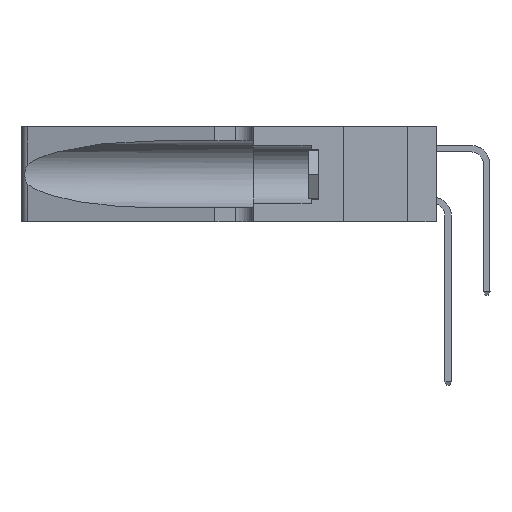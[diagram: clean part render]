
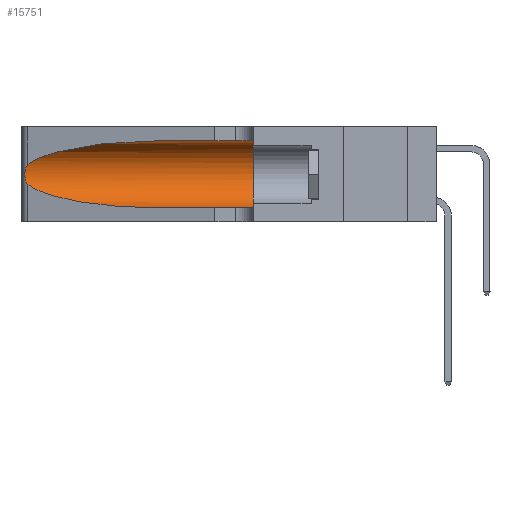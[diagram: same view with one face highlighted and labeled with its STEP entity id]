
A CAD part, left-side view. The second image highlights one B-rep face of the part: STEP entity #15751.
In plain terms, the highlighted cylindrical face has radius 3.308 mm (diameter 6.617 mm), a partial arc.
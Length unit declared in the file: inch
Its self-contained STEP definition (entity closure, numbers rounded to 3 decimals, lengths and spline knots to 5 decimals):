
#18 = DIRECTION ( 'NONE',  ( 0., -1., 0. ) ) ;
#241 = CARTESIAN_POINT ( 'NONE',  ( 0.1305, 0.35, 0.31525 ) ) ;
#1112 = ORIENTED_EDGE ( 'NONE', *, *, #20133, .T. ) ;
#1433 = VERTEX_POINT ( 'NONE', #8854 ) ;
#1655 = CARTESIAN_POINT ( 'NONE',  ( 0.25639, 1.23184, 0.21858 ) ) ;
#2651 = CARTESIAN_POINT ( 'NONE',  ( 0.1305, 0.35, 0.05475 ) ) ;
#3214 =( BOUNDED_CURVE ( )  B_SPLINE_CURVE ( 3, ( #38986, #42524, #31721, #24974 ),
 .UNSPECIFIED., .F., .F. ) 
 B_SPLINE_CURVE_WITH_KNOTS ( ( 4, 4 ),
 ( 1.5708, 2.84003 ),
 .UNSPECIFIED. ) 
 CURVE ( )  GEOMETRIC_REPRESENTATION_ITEM ( )  RATIONAL_B_SPLINE_CURVE ( ( 1., 0.87, 0.87, 1. ) ) 
 REPRESENTATION_ITEM ( '' )  );
#3647 = CARTESIAN_POINT ( 'NONE',  ( 0.1305, 1.61858, 0.185 ) ) ;
#5121 = VERTEX_POINT ( 'NONE', #241 ) ;
#5145 = EDGE_CURVE ( 'NONE', #41152, #26545, #39689, .T. ) ;
#5283 = CARTESIAN_POINT ( 'NONE',  ( 0.25854, 1.2359, 0.20912 ) ) ;
#7288 = AXIS2_PLACEMENT_3D ( 'NONE', #3647, #18, #17882 ) ;
#7499 = CARTESIAN_POINT ( 'NONE',  ( 0.25487, 1.22718, 0.22369 ) ) ;
#7794 = VERTEX_POINT ( 'NONE', #2651 ) ;
#8019 = VERTEX_POINT ( 'NONE', #7499 ) ;
#8032 = ORIENTED_EDGE ( 'NONE', *, *, #28097, .F. ) ;
#8177 = EDGE_CURVE ( 'NONE', #1433, #5121, #16339, .T. ) ;
#8854 = CARTESIAN_POINT ( 'NONE',  ( 0.1305, 0.72297, 0.31525 ) ) ;
#8910 = CARTESIAN_POINT ( 'NONE',  ( 0.26075, 1.23896, 0.19203 ) ) ;
#9117 = VECTOR ( 'NONE', #12959, 39.37008 ) ;
#9266 = FACE_OUTER_BOUND ( 'NONE', #29285, .T. ) ;
#9645 = ORIENTED_EDGE ( 'NONE', *, *, #5145, .T. ) ;
#10731 = AXIS2_PLACEMENT_3D ( 'NONE', #34669, #13424, #38259 ) ;
#11236 = CARTESIAN_POINT ( 'NONE',  ( 0.18966, 0.96281, 0.05475 ) ) ;
#11559 = B_SPLINE_CURVE_WITH_KNOTS ( 'NONE', 3,
 ( #40690, #15920, #1655, #26679, #5283, #30218, #8910, #33744, #12479, #37310, #16078, #40852, #19655, #44381 ),
 .UNSPECIFIED., .F., .F.,
 ( 4, 2, 2, 2, 2, 2, 4 ),
 ( 0., 0.00027, 0.00053, 0.00107, 0.0016, 0.00187, 0.00214 ),
 .UNSPECIFIED. ) ;
#12479 = CARTESIAN_POINT ( 'NONE',  ( 0.26017, 1.23833, 0.17102 ) ) ;
#12959 = DIRECTION ( 'NONE',  ( 0., -1., 0. ) ) ;
#13424 = DIRECTION ( 'NONE',  ( 0., 1., 0. ) ) ;
#14816 = CARTESIAN_POINT ( 'NONE',  ( 0.25487, 1.22718, 0.14631 ) ) ;
#15452 = CARTESIAN_POINT ( 'NONE',  ( 0.1305, 1.61858, 0.31525 ) ) ;
#15751 = ADVANCED_FACE ( 'NONE', ( #9266 ), #43611, .F. ) ;
#15920 = CARTESIAN_POINT ( 'NONE',  ( 0.25555, 1.22994, 0.2215 ) ) ;
#16078 = CARTESIAN_POINT ( 'NONE',  ( 0.25789, 1.23486, 0.15765 ) ) ;
#16339 = LINE ( 'NONE', #15452, #26951 ) ;
#16697 = CARTESIAN_POINT ( 'NONE',  ( 0.1305, 1.61858, 0.05475 ) ) ;
#17882 = DIRECTION ( 'NONE',  ( 0., 0., -1. ) ) ;
#18421 = CARTESIAN_POINT ( 'NONE',  ( 0.1305, 0.72297, 0.05475 ) ) ;
#19655 = CARTESIAN_POINT ( 'NONE',  ( 0.25555, 1.22993, 0.14849 ) ) ;
#20133 = EDGE_CURVE ( 'NONE', #26545, #7794, #37446, .T. ) ;
#20813 = ORIENTED_EDGE ( 'NONE', *, *, #28244, .T. ) ;
#24033 = CARTESIAN_POINT ( 'NONE',  ( 0.1305, 0.72297, 0.05475 ) ) ;
#24974 = CARTESIAN_POINT ( 'NONE',  ( 0.25487, 1.22718, 0.22369 ) ) ;
#26414 = EDGE_CURVE ( 'NONE', #8019, #41152, #11559, .T. ) ;
#26545 = VERTEX_POINT ( 'NONE', #24033 ) ;
#26679 = CARTESIAN_POINT ( 'NONE',  ( 0.25787, 1.23484, 0.2124 ) ) ;
#26951 = VECTOR ( 'NONE', #40225, 39.37008 ) ;
#28097 = EDGE_CURVE ( 'NONE', #5121, #7794, #36192, .T. ) ;
#28244 = EDGE_CURVE ( 'NONE', #1433, #8019, #3214, .T. ) ;
#29285 = EDGE_LOOP ( 'NONE', ( #20813, #37339, #9645, #1112, #8032, #32920 ) ) ;
#30218 = CARTESIAN_POINT ( 'NONE',  ( 0.26018, 1.23835, 0.19895 ) ) ;
#31721 = CARTESIAN_POINT ( 'NONE',  ( 0.2373, 1.15595, 0.28018 ) ) ;
#32920 = ORIENTED_EDGE ( 'NONE', *, *, #8177, .F. ) ;
#33744 = CARTESIAN_POINT ( 'NONE',  ( 0.26075, 1.23896, 0.178 ) ) ;
#34669 = CARTESIAN_POINT ( 'NONE',  ( 0.1305, 0.35, 0.185 ) ) ;
#36051 = CARTESIAN_POINT ( 'NONE',  ( 0.2373, 1.15595, 0.08982 ) ) ;
#36192 = CIRCLE ( 'NONE', #10731, 0.13025 ) ;
#37310 = CARTESIAN_POINT ( 'NONE',  ( 0.25856, 1.23593, 0.16098 ) ) ;
#37339 = ORIENTED_EDGE ( 'NONE', *, *, #26414, .T. ) ;
#37446 = LINE ( 'NONE', #16697, #9117 ) ;
#38259 = DIRECTION ( 'NONE',  ( 0., 0., 1. ) ) ;
#38986 = CARTESIAN_POINT ( 'NONE',  ( 0.1305, 0.72297, 0.31525 ) ) ;
#39689 =( BOUNDED_CURVE ( )  B_SPLINE_CURVE ( 3, ( #14816, #36051, #11236, #18421 ),
 .UNSPECIFIED., .F., .T. ) 
 B_SPLINE_CURVE_WITH_KNOTS ( ( 4, 4 ),
 ( 3.44316, 4.71239 ),
 .UNSPECIFIED. ) 
 CURVE ( )  GEOMETRIC_REPRESENTATION_ITEM ( )  RATIONAL_B_SPLINE_CURVE ( ( 1., 0.87, 0.87, 1. ) ) 
 REPRESENTATION_ITEM ( '' )  );
#40225 = DIRECTION ( 'NONE',  ( 0., -1., 0. ) ) ;
#40690 = CARTESIAN_POINT ( 'NONE',  ( 0.25487, 1.22718, 0.22369 ) ) ;
#40852 = CARTESIAN_POINT ( 'NONE',  ( 0.25639, 1.23186, 0.15144 ) ) ;
#41152 = VERTEX_POINT ( 'NONE', #42868 ) ;
#42524 = CARTESIAN_POINT ( 'NONE',  ( 0.18966, 0.96281, 0.31525 ) ) ;
#42868 = CARTESIAN_POINT ( 'NONE',  ( 0.25487, 1.22718, 0.14631 ) ) ;
#43611 = CYLINDRICAL_SURFACE ( 'NONE', #7288, 0.13025 ) ;
#44381 = CARTESIAN_POINT ( 'NONE',  ( 0.25487, 1.22718, 0.14631 ) ) ;
